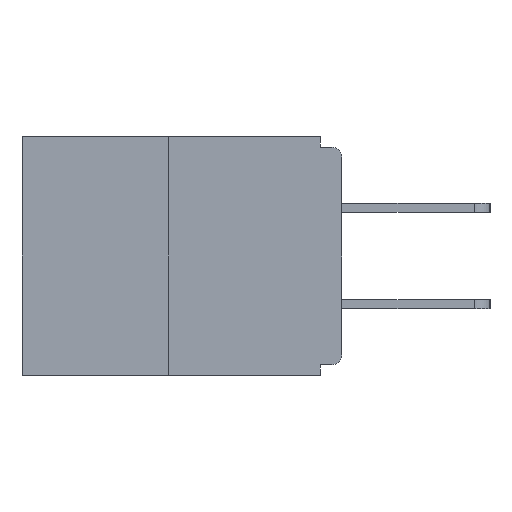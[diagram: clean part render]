
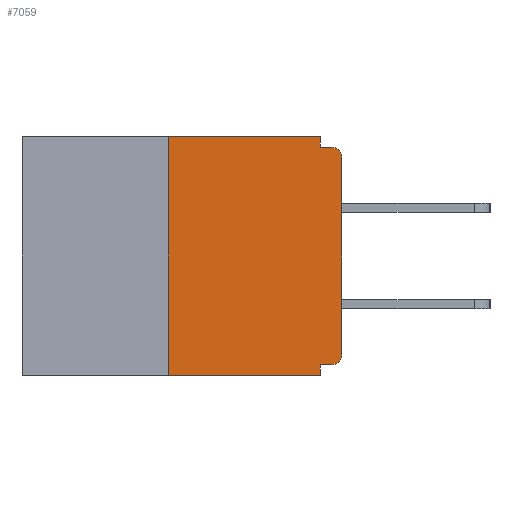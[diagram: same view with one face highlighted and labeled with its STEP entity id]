
A CAD part, left-side view. The second image highlights one B-rep face of the part: STEP entity #7059.
In plain terms, the highlighted planar face has unit normal (-1, 0, 0).
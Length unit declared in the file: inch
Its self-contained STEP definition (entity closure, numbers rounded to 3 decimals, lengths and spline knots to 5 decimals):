
#21 = VECTOR ( 'NONE', #5660, 39.37008 ) ;
#721 = DIRECTION ( 'NONE',  ( 0., 0., 1. ) ) ;
#849 = ORIENTED_EDGE ( 'NONE', *, *, #12254, .F. ) ;
#857 = EDGE_CURVE ( 'NONE', #2624, #8056, #18063, .T. ) ;
#943 = DIRECTION ( 'NONE',  ( -1., 0., 0. ) ) ;
#1185 = ORIENTED_EDGE ( 'NONE', *, *, #18609, .F. ) ;
#1204 = CARTESIAN_POINT ( 'NONE',  ( 0., 0.25, 0. ) ) ;
#1287 = VERTEX_POINT ( 'NONE', #14963 ) ;
#1930 = VECTOR ( 'NONE', #22332, 39.37008 ) ;
#2070 = VERTEX_POINT ( 'NONE', #17419 ) ;
#2624 = VERTEX_POINT ( 'NONE', #4973 ) ;
#4018 = CARTESIAN_POINT ( 'NONE',  ( 0., 0.46, -0.343 ) ) ;
#4063 = LINE ( 'NONE', #12549, #5096 ) ;
#4637 = LINE ( 'NONE', #19829, #9257 ) ;
#4973 = CARTESIAN_POINT ( 'NONE',  ( 0., 0.031, -0.328 ) ) ;
#5096 = VECTOR ( 'NONE', #6303, 39.37008 ) ;
#5630 = CARTESIAN_POINT ( 'NONE',  ( 0., 0.46, 0. ) ) ;
#5660 = DIRECTION ( 'NONE',  ( 0., 0., -1. ) ) ;
#5663 = ORIENTED_EDGE ( 'NONE', *, *, #14035, .F. ) ;
#6007 = AXIS2_PLACEMENT_3D ( 'NONE', #19421, #25253, #17035 ) ;
#6126 = LINE ( 'NONE', #4018, #13683 ) ;
#6180 = FACE_OUTER_BOUND ( 'NONE', #6452, .T. ) ;
#6303 = DIRECTION ( 'NONE',  ( 0., -1., 0. ) ) ;
#6452 = EDGE_LOOP ( 'NONE', ( #17453, #849, #18137, #15936, #5663, #11757, #24358, #23671, #1185, #27476 ) ) ;
#6661 = VERTEX_POINT ( 'NONE', #11557 ) ;
#6852 = EDGE_CURVE ( 'NONE', #1287, #11327, #15753, .T. ) ;
#6878 = EDGE_CURVE ( 'NONE', #14044, #11137, #27354, .T. ) ;
#7059 = ADVANCED_FACE ( 'NONE', ( #6180 ), #21503, .F. ) ;
#7247 = VERTEX_POINT ( 'NONE', #9484 ) ;
#7842 = DIRECTION ( 'NONE',  ( 0., 0., -1. ) ) ;
#8056 = VERTEX_POINT ( 'NONE', #24024 ) ;
#9257 = VECTOR ( 'NONE', #721, 39.37008 ) ;
#9484 = CARTESIAN_POINT ( 'NONE',  ( 0., 0.031, -0.015 ) ) ;
#9541 = CARTESIAN_POINT ( 'NONE',  ( 0., 0.031, -0.343 ) ) ;
#9555 = DIRECTION ( 'NONE',  ( 0., 0., -1. ) ) ;
#10278 = DIRECTION ( 'NONE',  ( 0., -1., 0. ) ) ;
#10339 = DIRECTION ( 'NONE',  ( 0., -1., 0. ) ) ;
#11137 = VERTEX_POINT ( 'NONE', #15160 ) ;
#11327 = VERTEX_POINT ( 'NONE', #25907 ) ;
#11557 = CARTESIAN_POINT ( 'NONE',  ( 0., 0., -0.313 ) ) ;
#11757 = ORIENTED_EDGE ( 'NONE', *, *, #27381, .T. ) ;
#11884 = DIRECTION ( 'NONE',  ( -1., 0., 0. ) ) ;
#12036 = AXIS2_PLACEMENT_3D ( 'NONE', #19643, #943, #15299 ) ;
#12254 = EDGE_CURVE ( 'NONE', #25842, #14044, #26791, .T. ) ;
#12549 = CARTESIAN_POINT ( 'NONE',  ( 0., 0., -0.015 ) ) ;
#13683 = VECTOR ( 'NONE', #10278, 39.37008 ) ;
#13772 = EDGE_CURVE ( 'NONE', #25842, #8056, #6126, .T. ) ;
#13792 = CARTESIAN_POINT ( 'NONE',  ( 0., 0.015, -0.03 ) ) ;
#14035 = EDGE_CURVE ( 'NONE', #2070, #2624, #23798, .T. ) ;
#14044 = VERTEX_POINT ( 'NONE', #1204 ) ;
#14101 = EDGE_CURVE ( 'NONE', #11137, #7247, #22114, .T. ) ;
#14118 = VECTOR ( 'NONE', #9555, 39.37008 ) ;
#14963 = CARTESIAN_POINT ( 'NONE',  ( 0., 0., -0.03 ) ) ;
#15160 = CARTESIAN_POINT ( 'NONE',  ( 0., 0.031, 0. ) ) ;
#15175 = CARTESIAN_POINT ( 'NONE',  ( 0., 0.25, -0.343 ) ) ;
#15299 = DIRECTION ( 'NONE',  ( 0., 0., -1. ) ) ;
#15329 = VECTOR ( 'NONE', #10339, 39.37008 ) ;
#15557 = DIRECTION ( 'NONE',  ( 0., 1., 0. ) ) ;
#15753 = CIRCLE ( 'NONE', #22890, 0.015 ) ;
#15906 = VECTOR ( 'NONE', #15557, 39.37008 ) ;
#15936 = ORIENTED_EDGE ( 'NONE', *, *, #857, .F. ) ;
#16111 = CARTESIAN_POINT ( 'NONE',  ( 0., 0.031, 0. ) ) ;
#17035 = DIRECTION ( 'NONE',  ( 0., 0., -1. ) ) ;
#17419 = CARTESIAN_POINT ( 'NONE',  ( 0., 0.015, -0.328 ) ) ;
#17453 = ORIENTED_EDGE ( 'NONE', *, *, #6878, .F. ) ;
#18063 = LINE ( 'NONE', #9541, #21 ) ;
#18137 = ORIENTED_EDGE ( 'NONE', *, *, #13772, .T. ) ;
#18609 = EDGE_CURVE ( 'NONE', #7247, #11327, #4063, .T. ) ;
#19421 = CARTESIAN_POINT ( 'NONE',  ( 0., 0.46, 0. ) ) ;
#19643 = CARTESIAN_POINT ( 'NONE',  ( 0., 0.015, -0.313 ) ) ;
#19829 = CARTESIAN_POINT ( 'NONE',  ( 0., 0., 0. ) ) ;
#20256 = CARTESIAN_POINT ( 'NONE',  ( 0., 0.25, 0. ) ) ;
#20417 = EDGE_CURVE ( 'NONE', #6661, #1287, #4637, .T. ) ;
#21503 = PLANE ( 'NONE',  #6007 ) ;
#21707 = CARTESIAN_POINT ( 'NONE',  ( 0., 0., -0.328 ) ) ;
#22114 = LINE ( 'NONE', #16111, #14118 ) ;
#22295 = CIRCLE ( 'NONE', #12036, 0.015 ) ;
#22332 = DIRECTION ( 'NONE',  ( 0., 0., 1. ) ) ;
#22890 = AXIS2_PLACEMENT_3D ( 'NONE', #13792, #11884, #7842 ) ;
#23671 = ORIENTED_EDGE ( 'NONE', *, *, #6852, .T. ) ;
#23798 = LINE ( 'NONE', #21707, #15906 ) ;
#24024 = CARTESIAN_POINT ( 'NONE',  ( 0., 0.031, -0.343 ) ) ;
#24358 = ORIENTED_EDGE ( 'NONE', *, *, #20417, .T. ) ;
#25253 = DIRECTION ( 'NONE',  ( 1., 0., 0. ) ) ;
#25842 = VERTEX_POINT ( 'NONE', #15175 ) ;
#25907 = CARTESIAN_POINT ( 'NONE',  ( 0., 0.015, -0.015 ) ) ;
#26791 = LINE ( 'NONE', #20256, #1930 ) ;
#27354 = LINE ( 'NONE', #5630, #15329 ) ;
#27381 = EDGE_CURVE ( 'NONE', #2070, #6661, #22295, .T. ) ;
#27476 = ORIENTED_EDGE ( 'NONE', *, *, #14101, .F. ) ;
